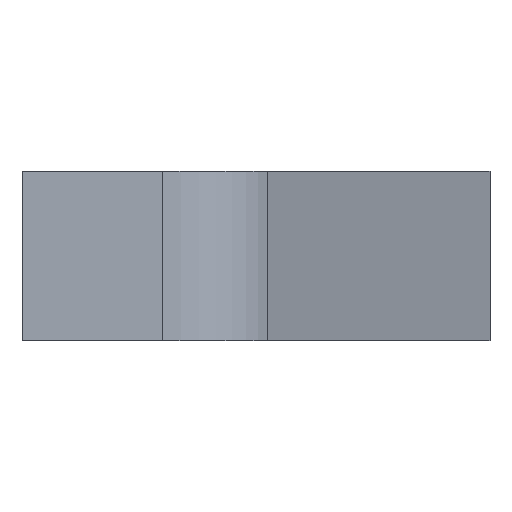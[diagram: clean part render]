
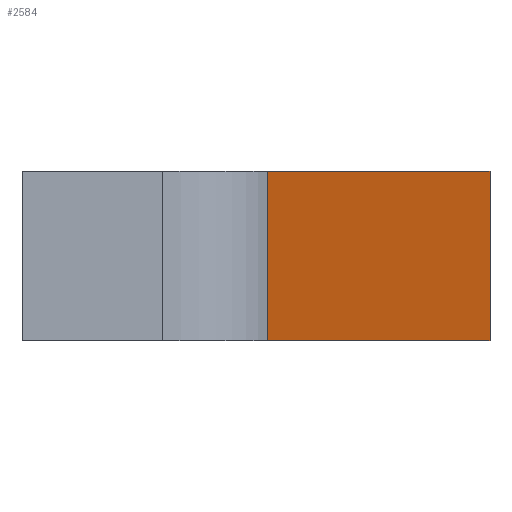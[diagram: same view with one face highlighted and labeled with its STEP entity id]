
A CAD part, left-side view. The second image highlights one B-rep face of the part: STEP entity #2584.
In plain terms, the highlighted planar face has unit normal (-0.437, -0.899, 0).
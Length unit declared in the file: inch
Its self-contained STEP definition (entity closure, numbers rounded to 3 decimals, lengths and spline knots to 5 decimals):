
#255 = ORIENTED_EDGE ( 'NONE', *, *, #2520, .F. ) ;
#295 = VERTEX_POINT ( 'NONE', #2959 ) ;
#454 = DIRECTION ( 'NONE',  ( 0.437, 0.899, 0. ) ) ;
#532 = CARTESIAN_POINT ( 'NONE',  ( 3.76036, 1.35286, 0.25009 ) ) ;
#635 = VECTOR ( 'NONE', #1322, 39.37008 ) ;
#761 = EDGE_CURVE ( 'NONE', #1898, #295, #3038, .T. ) ;
#843 = VERTEX_POINT ( 'NONE', #1227 ) ;
#892 = CARTESIAN_POINT ( 'NONE',  ( 3.02817, 1.70877, 1.51096 ) ) ;
#899 = VECTOR ( 'NONE', #1421, 39.37008 ) ;
#1130 = VECTOR ( 'NONE', #2711, 39.37008 ) ;
#1182 = DIRECTION ( 'NONE',  ( 0., 0., -1. ) ) ;
#1227 = CARTESIAN_POINT ( 'NONE',  ( 3.76036, 1.35286, 0.52209 ) ) ;
#1318 = DIRECTION ( 'NONE',  ( 0.899, -0.437, 0. ) ) ;
#1322 = DIRECTION ( 'NONE',  ( 0.899, -0.437, 0. ) ) ;
#1393 = LINE ( 'NONE', #2993, #635 ) ;
#1421 = DIRECTION ( 'NONE',  ( -0.899, 0.437, 0. ) ) ;
#1779 = CARTESIAN_POINT ( 'NONE',  ( 3.02817, 1.70877, 0.52209 ) ) ;
#1898 = VERTEX_POINT ( 'NONE', #1779 ) ;
#1942 = ORIENTED_EDGE ( 'NONE', *, *, #2092, .T. ) ;
#1975 = FACE_OUTER_BOUND ( 'NONE', #3268, .T. ) ;
#2055 = LINE ( 'NONE', #2272, #899 ) ;
#2092 = EDGE_CURVE ( 'NONE', #843, #1898, #2055, .T. ) ;
#2272 = CARTESIAN_POINT ( 'NONE',  ( 3.02817, 1.70877, 0.52209 ) ) ;
#2400 = LINE ( 'NONE', #3604, #1130 ) ;
#2421 = ORIENTED_EDGE ( 'NONE', *, *, #2476, .T. ) ;
#2427 = PLANE ( 'NONE',  #3329 ) ;
#2476 = EDGE_CURVE ( 'NONE', #295, #3447, #1393, .T. ) ;
#2520 = EDGE_CURVE ( 'NONE', #843, #3447, #2400, .T. ) ;
#2584 = ADVANCED_FACE ( 'NONE', ( #1975 ), #2427, .F. ) ;
#2711 = DIRECTION ( 'NONE',  ( 0., 0., -1. ) ) ;
#2875 = ORIENTED_EDGE ( 'NONE', *, *, #761, .T. ) ;
#2959 = CARTESIAN_POINT ( 'NONE',  ( 3.02817, 1.70877, 0.25009 ) ) ;
#2993 = CARTESIAN_POINT ( 'NONE',  ( 3.02817, 1.70877, 0.25009 ) ) ;
#3038 = LINE ( 'NONE', #892, #3351 ) ;
#3268 = EDGE_LOOP ( 'NONE', ( #1942, #2875, #2421, #255 ) ) ;
#3301 = CARTESIAN_POINT ( 'NONE',  ( 3.02817, 1.70877, 1.51096 ) ) ;
#3329 = AXIS2_PLACEMENT_3D ( 'NONE', #3301, #454, #1318 ) ;
#3351 = VECTOR ( 'NONE', #1182, 39.37008 ) ;
#3447 = VERTEX_POINT ( 'NONE', #532 ) ;
#3604 = CARTESIAN_POINT ( 'NONE',  ( 3.76036, 1.35286, 1.51096 ) ) ;
